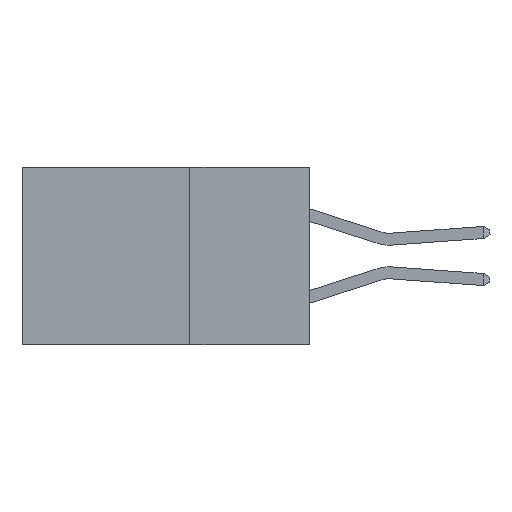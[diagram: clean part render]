
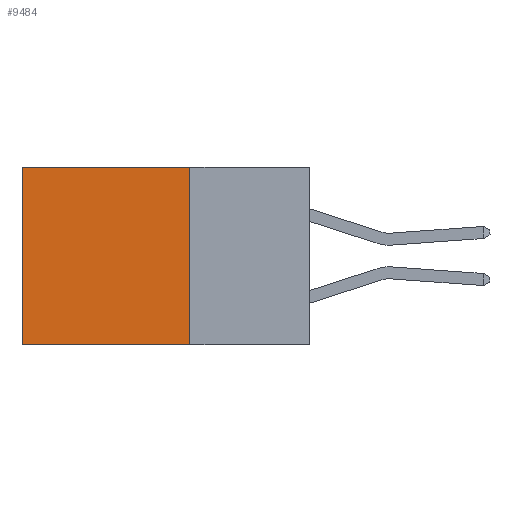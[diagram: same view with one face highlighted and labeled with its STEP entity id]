
A CAD part, left-side view. The second image highlights one B-rep face of the part: STEP entity #9484.
In plain terms, the highlighted planar face has unit normal (-1, 0, 0).
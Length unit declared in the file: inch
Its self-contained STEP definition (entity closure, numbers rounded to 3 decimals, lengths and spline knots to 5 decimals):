
#436 = CARTESIAN_POINT ( 'NONE',  ( 0.298, 0.25, 0. ) ) ;
#914 = ORIENTED_EDGE ( 'NONE', *, *, #934, .F. ) ;
#934 = EDGE_CURVE ( 'NONE', #4534, #2463, #2774, .T. ) ;
#1348 = CARTESIAN_POINT ( 'NONE',  ( 0.298, 0.25, 0. ) ) ;
#2463 = VERTEX_POINT ( 'NONE', #11091 ) ;
#2774 = LINE ( 'NONE', #436, #16380 ) ;
#2836 = ORIENTED_EDGE ( 'NONE', *, *, #7193, .F. ) ;
#2869 = CARTESIAN_POINT ( 'NONE',  ( 0.298, 0.6, 0. ) ) ;
#2924 = EDGE_LOOP ( 'NONE', ( #4609, #2836, #914, #12953 ) ) ;
#4534 = VERTEX_POINT ( 'NONE', #11942 ) ;
#4582 = VERTEX_POINT ( 'NONE', #10300 ) ;
#4609 = ORIENTED_EDGE ( 'NONE', *, *, #14872, .T. ) ;
#5520 = PLANE ( 'NONE',  #10384 ) ;
#6849 = DIRECTION ( 'NONE',  ( 1., 0., 0. ) ) ;
#6984 = CARTESIAN_POINT ( 'NONE',  ( 0.298, 0.25, -0.37 ) ) ;
#7193 = EDGE_CURVE ( 'NONE', #2463, #11931, #9924, .T. ) ;
#8568 = DIRECTION ( 'NONE',  ( 0., 0., -1. ) ) ;
#9421 = VECTOR ( 'NONE', #14697, 39.37008 ) ;
#9484 = ADVANCED_FACE ( 'NONE', ( #14811 ), #5520, .F. ) ;
#9848 = LINE ( 'NONE', #13209, #9421 ) ;
#9924 = LINE ( 'NONE', #6984, #16288 ) ;
#10300 = CARTESIAN_POINT ( 'NONE',  ( 0.298, 0.6, 0. ) ) ;
#10384 = AXIS2_PLACEMENT_3D ( 'NONE', #1348, #6849, #15957 ) ;
#10980 = DIRECTION ( 'NONE',  ( 0., 0., -1. ) ) ;
#11091 = CARTESIAN_POINT ( 'NONE',  ( 0.298, 0.25, -0.37 ) ) ;
#11931 = VERTEX_POINT ( 'NONE', #12641 ) ;
#11942 = CARTESIAN_POINT ( 'NONE',  ( 0.298, 0.25, 0. ) ) ;
#12641 = CARTESIAN_POINT ( 'NONE',  ( 0.298, 0.6, -0.37 ) ) ;
#12953 = ORIENTED_EDGE ( 'NONE', *, *, #14247, .T. ) ;
#13037 = LINE ( 'NONE', #2869, #15590 ) ;
#13209 = CARTESIAN_POINT ( 'NONE',  ( 0.298, 0.25, 0. ) ) ;
#14247 = EDGE_CURVE ( 'NONE', #4534, #4582, #9848, .T. ) ;
#14697 = DIRECTION ( 'NONE',  ( 0., 1., 0. ) ) ;
#14811 = FACE_OUTER_BOUND ( 'NONE', #2924, .T. ) ;
#14872 = EDGE_CURVE ( 'NONE', #4582, #11931, #13037, .T. ) ;
#15590 = VECTOR ( 'NONE', #10980, 39.37008 ) ;
#15957 = DIRECTION ( 'NONE',  ( 0., 0., -1. ) ) ;
#16288 = VECTOR ( 'NONE', #16902, 39.37008 ) ;
#16380 = VECTOR ( 'NONE', #8568, 39.37008 ) ;
#16902 = DIRECTION ( 'NONE',  ( 0., 1., 0. ) ) ;
